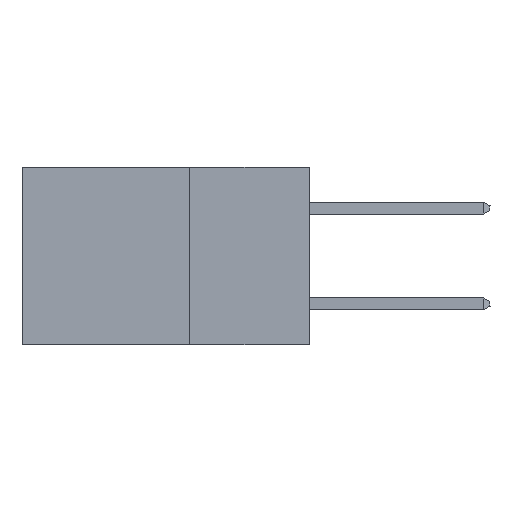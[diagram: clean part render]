
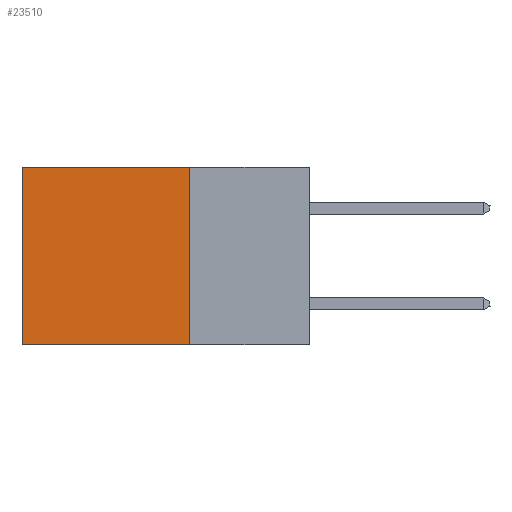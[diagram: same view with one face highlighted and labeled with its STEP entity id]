
A CAD part, left-side view. The second image highlights one B-rep face of the part: STEP entity #23510.
In plain terms, the highlighted planar face has unit normal (-1, 0, 0).
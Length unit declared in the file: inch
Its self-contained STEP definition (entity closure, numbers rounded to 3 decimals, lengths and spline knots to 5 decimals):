
#414 = DIRECTION ( 'NONE',  ( 0., 0., -1. ) ) ;
#5358 = FACE_OUTER_BOUND ( 'NONE', #23168, .T. ) ;
#6605 = DIRECTION ( 'NONE',  ( 1., 0., 0. ) ) ;
#6819 = VERTEX_POINT ( 'NONE', #43142 ) ;
#7201 = DIRECTION ( 'NONE',  ( 0., 0., -1. ) ) ;
#7541 = CARTESIAN_POINT ( 'NONE',  ( 0.2875, 0.25, 0. ) ) ;
#8917 = ORIENTED_EDGE ( 'NONE', *, *, #18198, .F. ) ;
#9979 = CARTESIAN_POINT ( 'NONE',  ( 0.2875, 0.25, 0. ) ) ;
#12046 = VERTEX_POINT ( 'NONE', #40433 ) ;
#12612 = CARTESIAN_POINT ( 'NONE',  ( 0.2875, 0.25, -0.37 ) ) ;
#14383 = DIRECTION ( 'NONE',  ( 0., 1., 0. ) ) ;
#14390 = AXIS2_PLACEMENT_3D ( 'NONE', #34906, #6605, #7201 ) ;
#15020 = VECTOR ( 'NONE', #19809, 39.37008 ) ;
#16742 = ORIENTED_EDGE ( 'NONE', *, *, #33073, .F. ) ;
#17578 = PLANE ( 'NONE',  #14390 ) ;
#18083 = CARTESIAN_POINT ( 'NONE',  ( 0.2875, 0.25, 0. ) ) ;
#18198 = EDGE_CURVE ( 'NONE', #12046, #6819, #24367, .T. ) ;
#19030 = ORIENTED_EDGE ( 'NONE', *, *, #37207, .T. ) ;
#19039 = VECTOR ( 'NONE', #43071, 39.37008 ) ;
#19479 = VERTEX_POINT ( 'NONE', #9979 ) ;
#19809 = DIRECTION ( 'NONE',  ( 0., 1., 0. ) ) ;
#23168 = EDGE_LOOP ( 'NONE', ( #40420, #8917, #16742, #19030 ) ) ;
#23510 = ADVANCED_FACE ( 'NONE', ( #5358 ), #17578, .F. ) ;
#24367 = LINE ( 'NONE', #12612, #15020 ) ;
#24654 = CARTESIAN_POINT ( 'NONE',  ( 0.2875, 0.6, 0. ) ) ;
#31849 = VERTEX_POINT ( 'NONE', #24654 ) ;
#33073 = EDGE_CURVE ( 'NONE', #19479, #12046, #37344, .T. ) ;
#33676 = LINE ( 'NONE', #36091, #39812 ) ;
#34906 = CARTESIAN_POINT ( 'NONE',  ( 0.2875, 0.25, 0. ) ) ;
#36091 = CARTESIAN_POINT ( 'NONE',  ( 0.2875, 0.6, 0. ) ) ;
#37207 = EDGE_CURVE ( 'NONE', #19479, #31849, #39167, .T. ) ;
#37344 = LINE ( 'NONE', #18083, #19039 ) ;
#38564 = EDGE_CURVE ( 'NONE', #31849, #6819, #33676, .T. ) ;
#39167 = LINE ( 'NONE', #7541, #45874 ) ;
#39812 = VECTOR ( 'NONE', #414, 39.37008 ) ;
#40420 = ORIENTED_EDGE ( 'NONE', *, *, #38564, .T. ) ;
#40433 = CARTESIAN_POINT ( 'NONE',  ( 0.2875, 0.25, -0.37 ) ) ;
#43071 = DIRECTION ( 'NONE',  ( 0., 0., -1. ) ) ;
#43142 = CARTESIAN_POINT ( 'NONE',  ( 0.2875, 0.6, -0.37 ) ) ;
#45874 = VECTOR ( 'NONE', #14383, 39.37008 ) ;
